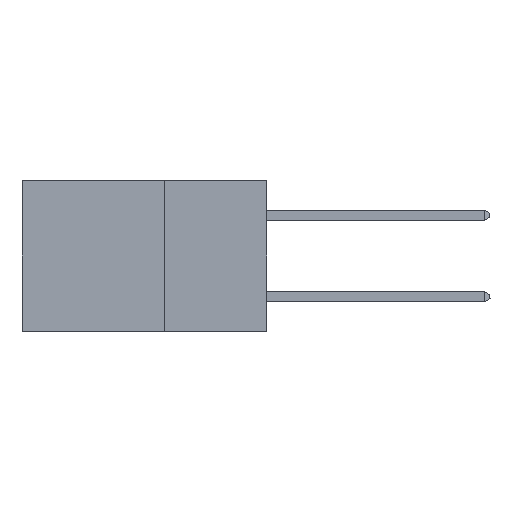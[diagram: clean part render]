
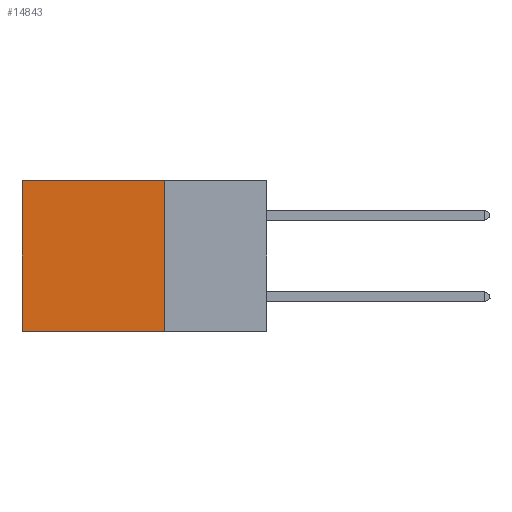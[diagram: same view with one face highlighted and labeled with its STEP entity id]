
A CAD part, left-side view. The second image highlights one B-rep face of the part: STEP entity #14843.
In plain terms, the highlighted planar face has unit normal (-1, 0, 0).
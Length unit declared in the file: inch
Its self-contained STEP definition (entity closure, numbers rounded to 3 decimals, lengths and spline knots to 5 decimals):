
#63 = ORIENTED_EDGE ( 'NONE', *, *, #6033, .T. ) ;
#302 = LINE ( 'NONE', #12194, #8177 ) ;
#627 = VECTOR ( 'NONE', #14007, 39.37008 ) ;
#809 = VERTEX_POINT ( 'NONE', #8263 ) ;
#1359 = VECTOR ( 'NONE', #10542, 39.37008 ) ;
#1761 = CARTESIAN_POINT ( 'NONE',  ( 0.2875, 0.25, 0. ) ) ;
#2973 = VERTEX_POINT ( 'NONE', #5443 ) ;
#5123 = EDGE_CURVE ( 'NONE', #809, #2973, #21234, .T. ) ;
#5443 = CARTESIAN_POINT ( 'NONE',  ( 0.2875, 0.6, 0. ) ) ;
#5775 = CARTESIAN_POINT ( 'NONE',  ( 0.2875, 0.6, 0. ) ) ;
#5818 = LINE ( 'NONE', #22597, #1359 ) ;
#5874 = VERTEX_POINT ( 'NONE', #13561 ) ;
#5909 = DIRECTION ( 'NONE',  ( 1., 0., 0. ) ) ;
#6033 = EDGE_CURVE ( 'NONE', #2973, #5874, #15945, .T. ) ;
#7821 = ORIENTED_EDGE ( 'NONE', *, *, #18845, .F. ) ;
#8177 = VECTOR ( 'NONE', #22205, 39.37008 ) ;
#8263 = CARTESIAN_POINT ( 'NONE',  ( 0.2875, 0.25, 0. ) ) ;
#9907 = CARTESIAN_POINT ( 'NONE',  ( 0.2875, 0.25, 0. ) ) ;
#10542 = DIRECTION ( 'NONE',  ( 0., 1., 0. ) ) ;
#11435 = AXIS2_PLACEMENT_3D ( 'NONE', #1761, #5909, #19751 ) ;
#12194 = CARTESIAN_POINT ( 'NONE',  ( 0.2875, 0.25, 0. ) ) ;
#13561 = CARTESIAN_POINT ( 'NONE',  ( 0.2875, 0.6, -0.37 ) ) ;
#14007 = DIRECTION ( 'NONE',  ( 0., 0., -1. ) ) ;
#14347 = EDGE_CURVE ( 'NONE', #21852, #5874, #5818, .T. ) ;
#14843 = ADVANCED_FACE ( 'NONE', ( #22463 ), #25525, .F. ) ;
#15679 = ORIENTED_EDGE ( 'NONE', *, *, #14347, .F. ) ;
#15885 = DIRECTION ( 'NONE',  ( 0., 1., 0. ) ) ;
#15945 = LINE ( 'NONE', #5775, #627 ) ;
#18845 = EDGE_CURVE ( 'NONE', #809, #21852, #302, .T. ) ;
#19751 = DIRECTION ( 'NONE',  ( 0., 0., -1. ) ) ;
#20437 = CARTESIAN_POINT ( 'NONE',  ( 0.2875, 0.25, -0.37 ) ) ;
#21234 = LINE ( 'NONE', #9907, #22761 ) ;
#21852 = VERTEX_POINT ( 'NONE', #20437 ) ;
#22205 = DIRECTION ( 'NONE',  ( 0., 0., -1. ) ) ;
#22463 = FACE_OUTER_BOUND ( 'NONE', #25063, .T. ) ;
#22597 = CARTESIAN_POINT ( 'NONE',  ( 0.2875, 0.25, -0.37 ) ) ;
#22761 = VECTOR ( 'NONE', #15885, 39.37008 ) ;
#24949 = ORIENTED_EDGE ( 'NONE', *, *, #5123, .T. ) ;
#25063 = EDGE_LOOP ( 'NONE', ( #63, #15679, #7821, #24949 ) ) ;
#25525 = PLANE ( 'NONE',  #11435 ) ;
